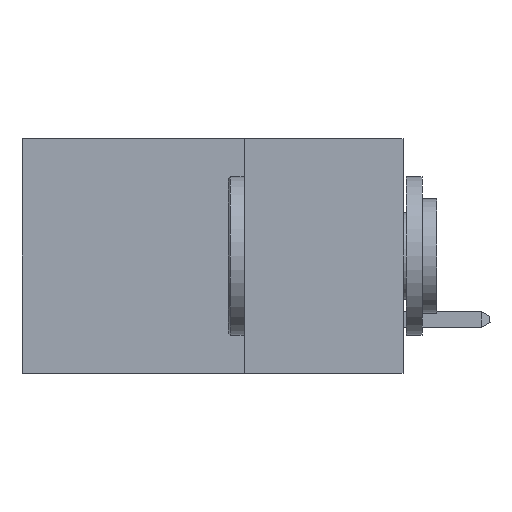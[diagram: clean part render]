
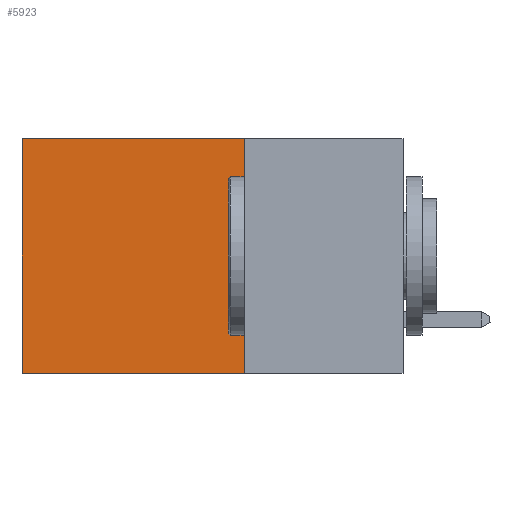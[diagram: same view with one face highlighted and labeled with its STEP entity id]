
A CAD part, left-side view. The second image highlights one B-rep face of the part: STEP entity #5923.
In plain terms, the highlighted planar face has unit normal (-1, 0, 0).
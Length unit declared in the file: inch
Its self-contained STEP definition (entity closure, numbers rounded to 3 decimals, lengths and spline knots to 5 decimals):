
#103 = FACE_OUTER_BOUND ( 'NONE', #26936, .T. ) ;
#5047 = CARTESIAN_POINT ( 'NONE',  ( 0.2875, 0.25, 0. ) ) ;
#5923 = ADVANCED_FACE ( 'NONE', ( #103 ), #40694, .F. ) ;
#6008 = CARTESIAN_POINT ( 'NONE',  ( 0.2875, 0.6, 0. ) ) ;
#6083 = CARTESIAN_POINT ( 'NONE',  ( 0.2875, 0.25, -0.37 ) ) ;
#6986 = ORIENTED_EDGE ( 'NONE', *, *, #19369, .T. ) ;
#8893 = VECTOR ( 'NONE', #44905, 39.37008 ) ;
#9307 = ORIENTED_EDGE ( 'NONE', *, *, #16975, .T. ) ;
#9923 = DIRECTION ( 'NONE',  ( 0., 1., 0. ) ) ;
#9996 = VERTEX_POINT ( 'NONE', #6008 ) ;
#12228 = CARTESIAN_POINT ( 'NONE',  ( 0.2875, 0.25, -0.37 ) ) ;
#13570 = CARTESIAN_POINT ( 'NONE',  ( 0.2875, 0.6, 0. ) ) ;
#15753 = EDGE_CURVE ( 'NONE', #19826, #38376, #39572, .T. ) ;
#16517 = DIRECTION ( 'NONE',  ( 0., 1., 0. ) ) ;
#16975 = EDGE_CURVE ( 'NONE', #9996, #38376, #21147, .T. ) ;
#17175 = VECTOR ( 'NONE', #16517, 39.37008 ) ;
#19369 = EDGE_CURVE ( 'NONE', #23864, #9996, #23188, .T. ) ;
#19394 = CARTESIAN_POINT ( 'NONE',  ( 0.2875, 0.25, 0. ) ) ;
#19826 = VERTEX_POINT ( 'NONE', #12228 ) ;
#21147 = LINE ( 'NONE', #13570, #42457 ) ;
#22062 = VECTOR ( 'NONE', #9923, 39.37008 ) ;
#23188 = LINE ( 'NONE', #35012, #22062 ) ;
#23240 = ORIENTED_EDGE ( 'NONE', *, *, #15753, .F. ) ;
#23864 = VERTEX_POINT ( 'NONE', #31423 ) ;
#24527 = DIRECTION ( 'NONE',  ( 0., 0., -1. ) ) ;
#26267 = EDGE_CURVE ( 'NONE', #23864, #19826, #44203, .T. ) ;
#26633 = ORIENTED_EDGE ( 'NONE', *, *, #26267, .F. ) ;
#26936 = EDGE_LOOP ( 'NONE', ( #9307, #23240, #26633, #6986 ) ) ;
#29893 = DIRECTION ( 'NONE',  ( 0., 0., -1. ) ) ;
#30367 = DIRECTION ( 'NONE',  ( 1., 0., 0. ) ) ;
#31423 = CARTESIAN_POINT ( 'NONE',  ( 0.2875, 0.25, 0. ) ) ;
#35012 = CARTESIAN_POINT ( 'NONE',  ( 0.2875, 0.25, 0. ) ) ;
#35819 = CARTESIAN_POINT ( 'NONE',  ( 0.2875, 0.6, -0.37 ) ) ;
#35986 = AXIS2_PLACEMENT_3D ( 'NONE', #19394, #30367, #29893 ) ;
#38376 = VERTEX_POINT ( 'NONE', #35819 ) ;
#39572 = LINE ( 'NONE', #6083, #17175 ) ;
#40694 = PLANE ( 'NONE',  #35986 ) ;
#42457 = VECTOR ( 'NONE', #24527, 39.37008 ) ;
#44203 = LINE ( 'NONE', #5047, #8893 ) ;
#44905 = DIRECTION ( 'NONE',  ( 0., 0., -1. ) ) ;
